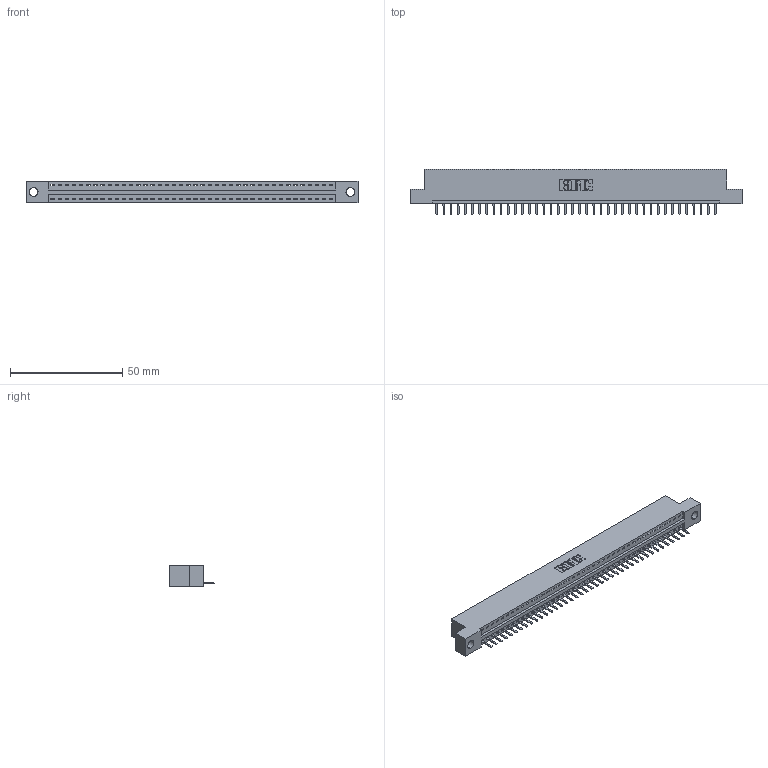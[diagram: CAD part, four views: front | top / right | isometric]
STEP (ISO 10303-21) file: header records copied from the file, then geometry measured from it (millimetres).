
FILE_DESCRIPTION (( 'STEP AP203' ), '1' );
FILE_NAME ('346-040-520-104.STEP', '2018-08-24T08:19:13', ( '' ), ( '' ), 'SwSTEP 2.0', 'SolidWorks 2016', '' );
FILE_SCHEMA (( 'CONFIG_CONTROL_DESIGN' ));
Length unit declared in the file: inch
Products named in the file (3): 346 Part_Flush Mounting Lugs - 0.156 Dia-TH; 345-292-001_345-293-120; 346-040-520-104
Assembly tree (41 placements, depth 2):
  346-040-520-104
    346 Part_Flush Mounting Lugs - 0.156 Dia-TH
    345-292-001_345-293-120  x40
Bounding box: 147.57 x 20.02 x 9.4 mm (x, y, z)
Volume: 13909.4 mm3; surface area: 16784.3 mm2
Topology: 41 solids, 41 shells, 2602 faces, 7689 edges, 5018 vertices
Faces by surface type: plane 1756, cylinder 846
Entity records: 25211 total; most frequent: CARTESIAN_POINT 4340, ORIENTED_EDGE 4302, DIRECTION 3819, EDGE_CURVE 2151, LINE 1855, VECTOR 1855, VERTEX_POINT 1430, AXIS2_PLACEMENT_3D 982
